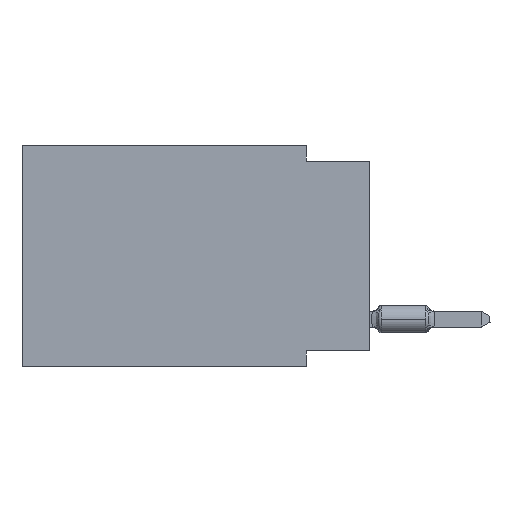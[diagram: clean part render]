
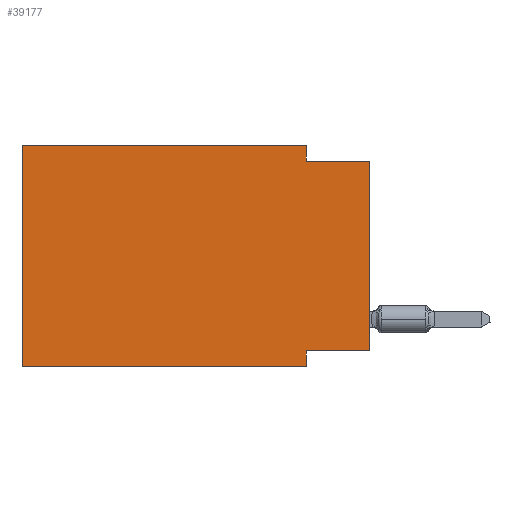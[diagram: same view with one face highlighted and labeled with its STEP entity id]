
A CAD part, left-side view. The second image highlights one B-rep face of the part: STEP entity #39177.
In plain terms, the highlighted planar face has unit normal (-1, 0, 0).
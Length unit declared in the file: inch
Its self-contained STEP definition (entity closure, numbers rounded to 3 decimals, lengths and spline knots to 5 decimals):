
#3220 = VERTEX_POINT ( 'NONE', #46993 ) ;
#3364 = ORIENTED_EDGE ( 'NONE', *, *, #48824, .F. ) ;
#4964 = CARTESIAN_POINT ( 'NONE',  ( 0., 0., 0. ) ) ;
#5484 = VERTEX_POINT ( 'NONE', #47301 ) ;
#7537 = VERTEX_POINT ( 'NONE', #105357 ) ;
#10762 = CARTESIAN_POINT ( 'NONE',  ( 0., 0.1, -0.025 ) ) ;
#11069 = VECTOR ( 'NONE', #109177, 39.37008 ) ;
#13802 = DIRECTION ( 'NONE',  ( 0., 0., 1. ) ) ;
#17875 = ORIENTED_EDGE ( 'NONE', *, *, #104357, .F. ) ;
#23741 = VECTOR ( 'NONE', #75146, 39.37008 ) ;
#26648 = ORIENTED_EDGE ( 'NONE', *, *, #108601, .F. ) ;
#27651 = CARTESIAN_POINT ( 'NONE',  ( 0., 0.55, -0.35 ) ) ;
#28160 = CARTESIAN_POINT ( 'NONE',  ( 0., 0.55, 0. ) ) ;
#30477 = DIRECTION ( 'NONE',  ( 0., -1., 0. ) ) ;
#32011 = DIRECTION ( 'NONE',  ( 0., 0., 1. ) ) ;
#32830 = VECTOR ( 'NONE', #101095, 39.37008 ) ;
#36998 = VERTEX_POINT ( 'NONE', #40900 ) ;
#39177 = ADVANCED_FACE ( 'NONE', ( #100451 ), #91043, .F. ) ;
#40900 = CARTESIAN_POINT ( 'NONE',  ( 0., 0.1, 0. ) ) ;
#42677 = DIRECTION ( 'NONE',  ( 0., 0., -1. ) ) ;
#44238 = CARTESIAN_POINT ( 'NONE',  ( 0., 0.55, -0.35 ) ) ;
#46378 = CARTESIAN_POINT ( 'NONE',  ( 0., 0., -0.025 ) ) ;
#46430 = EDGE_CURVE ( 'NONE', #68395, #7537, #58489, .T. ) ;
#46993 = CARTESIAN_POINT ( 'NONE',  ( 0., 0., -0.325 ) ) ;
#47301 = CARTESIAN_POINT ( 'NONE',  ( 0., 0.1, -0.35 ) ) ;
#47841 = VECTOR ( 'NONE', #32011, 39.37008 ) ;
#48824 = EDGE_CURVE ( 'NONE', #98800, #67970, #110448, .T. ) ;
#49990 = ORIENTED_EDGE ( 'NONE', *, *, #107785, .F. ) ;
#50207 = LINE ( 'NONE', #4964, #47841 ) ;
#55083 = CARTESIAN_POINT ( 'NONE',  ( 0., 0., -0.325 ) ) ;
#57256 = VECTOR ( 'NONE', #30477, 39.37008 ) ;
#58489 = LINE ( 'NONE', #94323, #100384 ) ;
#59454 = VERTEX_POINT ( 'NONE', #67911 ) ;
#61851 = ORIENTED_EDGE ( 'NONE', *, *, #72933, .T. ) ;
#63354 = LINE ( 'NONE', #55083, #11069 ) ;
#65194 = DIRECTION ( 'NONE',  ( 0., 0., -1. ) ) ;
#66853 = CARTESIAN_POINT ( 'NONE',  ( 0., 0.1, -0.35 ) ) ;
#67911 = CARTESIAN_POINT ( 'NONE',  ( 0., 0.1, -0.325 ) ) ;
#67970 = VERTEX_POINT ( 'NONE', #98433 ) ;
#68395 = VERTEX_POINT ( 'NONE', #44238 ) ;
#68628 = LINE ( 'NONE', #111569, #23741 ) ;
#69432 = CARTESIAN_POINT ( 'NONE',  ( 0., 0.1, 0. ) ) ;
#69529 = ORIENTED_EDGE ( 'NONE', *, *, #97595, .T. ) ;
#72933 = EDGE_CURVE ( 'NONE', #3220, #67970, #50207, .T. ) ;
#75066 = ORIENTED_EDGE ( 'NONE', *, *, #75423, .F. ) ;
#75146 = DIRECTION ( 'NONE',  ( 0., -1., 0. ) ) ;
#75299 = VECTOR ( 'NONE', #42677, 39.37008 ) ;
#75423 = EDGE_CURVE ( 'NONE', #7537, #36998, #68628, .T. ) ;
#78242 = LINE ( 'NONE', #69432, #101510 ) ;
#84551 = DIRECTION ( 'NONE',  ( 1., 0., 0. ) ) ;
#87330 = EDGE_LOOP ( 'NONE', ( #61851, #3364, #49990, #75066, #98425, #69529, #26648, #17875 ) ) ;
#87356 = LINE ( 'NONE', #66853, #75299 ) ;
#91043 = PLANE ( 'NONE',  #107731 ) ;
#94323 = CARTESIAN_POINT ( 'NONE',  ( 0., 0.55, 0. ) ) ;
#97595 = EDGE_CURVE ( 'NONE', #68395, #5484, #108206, .T. ) ;
#98425 = ORIENTED_EDGE ( 'NONE', *, *, #46430, .F. ) ;
#98433 = CARTESIAN_POINT ( 'NONE',  ( 0., 0., -0.025 ) ) ;
#98800 = VERTEX_POINT ( 'NONE', #10762 ) ;
#100384 = VECTOR ( 'NONE', #13802, 39.37008 ) ;
#100451 = FACE_OUTER_BOUND ( 'NONE', #87330, .T. ) ;
#101095 = DIRECTION ( 'NONE',  ( 0., -1., 0. ) ) ;
#101510 = VECTOR ( 'NONE', #105283, 39.37008 ) ;
#104357 = EDGE_CURVE ( 'NONE', #3220, #59454, #63354, .T. ) ;
#105283 = DIRECTION ( 'NONE',  ( 0., 0., -1. ) ) ;
#105357 = CARTESIAN_POINT ( 'NONE',  ( 0., 0.55, 0. ) ) ;
#107731 = AXIS2_PLACEMENT_3D ( 'NONE', #28160, #84551, #65194 ) ;
#107785 = EDGE_CURVE ( 'NONE', #36998, #98800, #78242, .T. ) ;
#108206 = LINE ( 'NONE', #27651, #32830 ) ;
#108601 = EDGE_CURVE ( 'NONE', #59454, #5484, #87356, .T. ) ;
#109177 = DIRECTION ( 'NONE',  ( 0., 1., 0. ) ) ;
#110448 = LINE ( 'NONE', #46378, #57256 ) ;
#111569 = CARTESIAN_POINT ( 'NONE',  ( 0., 0.55, 0. ) ) ;
